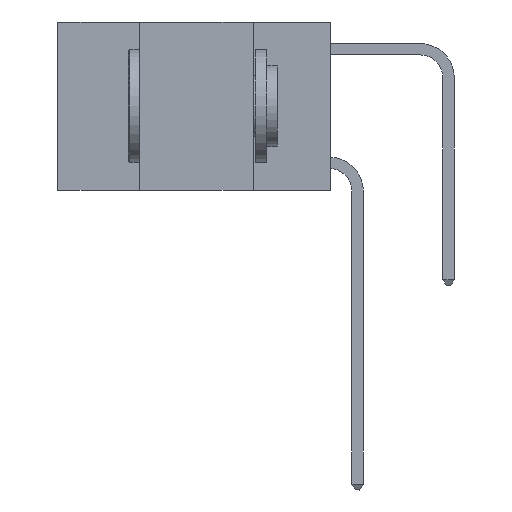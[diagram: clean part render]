
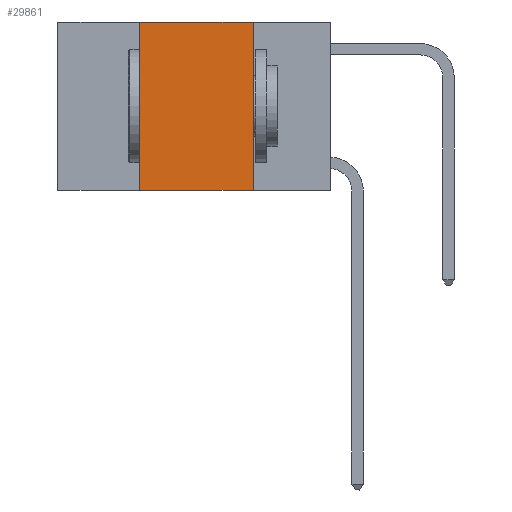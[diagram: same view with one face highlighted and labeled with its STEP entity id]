
A CAD part, left-side view. The second image highlights one B-rep face of the part: STEP entity #29861.
In plain terms, the highlighted planar face has unit normal (-1, 0, 0).
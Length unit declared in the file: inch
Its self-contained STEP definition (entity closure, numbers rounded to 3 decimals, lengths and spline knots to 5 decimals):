
#1346 = EDGE_CURVE ( 'NONE', #10161, #16344, #2035, .T. ) ;
#1749 = DIRECTION ( 'NONE',  ( 0., 0., -1. ) ) ;
#2035 = LINE ( 'NONE', #13247, #11488 ) ;
#2596 = ORIENTED_EDGE ( 'NONE', *, *, #1346, .F. ) ;
#4006 = LINE ( 'NONE', #20348, #15589 ) ;
#4193 = DIRECTION ( 'NONE',  ( 0., 0., 1. ) ) ;
#5080 = VECTOR ( 'NONE', #10827, 39.37008 ) ;
#5384 = CARTESIAN_POINT ( 'NONE',  ( 0., 0.6, -0.37 ) ) ;
#5661 = EDGE_CURVE ( 'NONE', #18227, #16344, #16904, .T. ) ;
#8960 = ORIENTED_EDGE ( 'NONE', *, *, #5661, .T. ) ;
#9440 = AXIS2_PLACEMENT_3D ( 'NONE', #13334, #22583, #18468 ) ;
#10161 = VERTEX_POINT ( 'NONE', #27116 ) ;
#10389 = VERTEX_POINT ( 'NONE', #14511 ) ;
#10827 = DIRECTION ( 'NONE',  ( 0., -1., 0. ) ) ;
#10989 = EDGE_CURVE ( 'NONE', #10389, #10161, #4006, .T. ) ;
#11488 = VECTOR ( 'NONE', #1749, 39.37008 ) ;
#13247 = CARTESIAN_POINT ( 'NONE',  ( 0., 0.17, 0. ) ) ;
#13334 = CARTESIAN_POINT ( 'NONE',  ( 0., 0.6, 0. ) ) ;
#13487 = FACE_OUTER_BOUND ( 'NONE', #21459, .T. ) ;
#14511 = CARTESIAN_POINT ( 'NONE',  ( 0., 0.42, 0. ) ) ;
#15210 = DIRECTION ( 'NONE',  ( 0., -1., 0. ) ) ;
#15589 = VECTOR ( 'NONE', #15210, 39.37008 ) ;
#15695 = LINE ( 'NONE', #24953, #21591 ) ;
#16344 = VERTEX_POINT ( 'NONE', #29747 ) ;
#16904 = LINE ( 'NONE', #5384, #5080 ) ;
#17215 = EDGE_CURVE ( 'NONE', #18227, #10389, #15695, .T. ) ;
#18227 = VERTEX_POINT ( 'NONE', #25773 ) ;
#18468 = DIRECTION ( 'NONE',  ( 0., 0., -1. ) ) ;
#18907 = ORIENTED_EDGE ( 'NONE', *, *, #17215, .F. ) ;
#20291 = PLANE ( 'NONE',  #9440 ) ;
#20348 = CARTESIAN_POINT ( 'NONE',  ( 0., 0.6, 0. ) ) ;
#21459 = EDGE_LOOP ( 'NONE', ( #2596, #27299, #18907, #8960 ) ) ;
#21591 = VECTOR ( 'NONE', #4193, 39.37008 ) ;
#22583 = DIRECTION ( 'NONE',  ( 1., 0., 0. ) ) ;
#24953 = CARTESIAN_POINT ( 'NONE',  ( 0., 0.42, 0. ) ) ;
#25773 = CARTESIAN_POINT ( 'NONE',  ( 0., 0.42, -0.37 ) ) ;
#27116 = CARTESIAN_POINT ( 'NONE',  ( 0., 0.17, 0. ) ) ;
#27299 = ORIENTED_EDGE ( 'NONE', *, *, #10989, .F. ) ;
#29747 = CARTESIAN_POINT ( 'NONE',  ( 0., 0.17, -0.37 ) ) ;
#29861 = ADVANCED_FACE ( 'NONE', ( #13487 ), #20291, .F. ) ;
